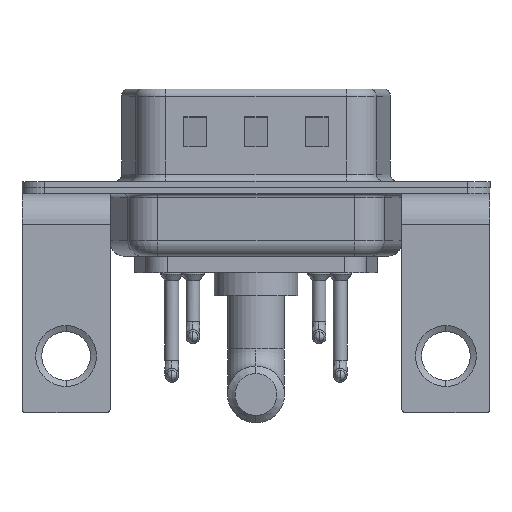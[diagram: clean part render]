
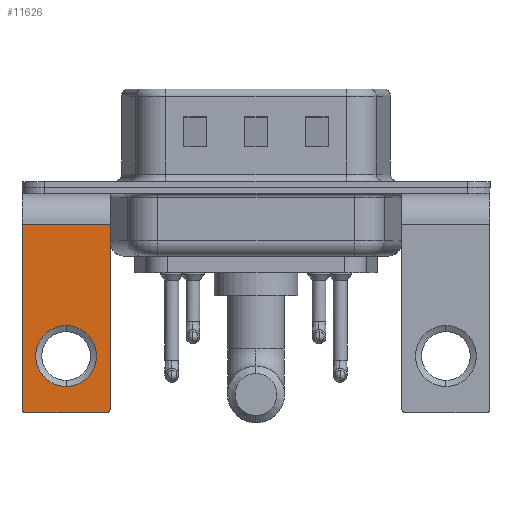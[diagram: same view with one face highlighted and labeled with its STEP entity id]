
A CAD part, front view. The second image highlights one B-rep face of the part: STEP entity #11626.
In plain terms, the highlighted planar face has unit normal (0, -1, 0).
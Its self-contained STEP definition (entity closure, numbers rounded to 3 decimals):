
#47 = EDGE_CURVE ( 'NONE', #15634, #13365, #19505, .T. ) ;
#176 = EDGE_CURVE ( 'NONE', #12546, #8315, #11063, .T. ) ;
#323 = ORIENTED_EDGE ( 'NONE', *, *, #14490, .F. ) ;
#403 = DIRECTION ( 'NONE',  ( 0., 0., 1. ) ) ;
#641 = DIRECTION ( 'NONE',  ( 0., 0., 1. ) ) ;
#1156 = AXIS2_PLACEMENT_3D ( 'NONE', #2812, #17855, #3937 ) ;
#1226 = PLANE ( 'NONE',  #7671 ) ;
#1314 = ORIENTED_EDGE ( 'NONE', *, *, #11258, .T. ) ;
#1354 = CARTESIAN_POINT ( 'NONE',  ( 0., -6.25, -9.07 ) ) ;
#2005 = CARTESIAN_POINT ( 'NONE',  ( 2.9, -6.25, -14.55 ) ) ;
#2027 = LINE ( 'NONE', #19199, #3482 ) ;
#2284 = VERTEX_POINT ( 'NONE', #2005 ) ;
#2810 = CIRCLE ( 'NONE', #13522, 0.25 ) ;
#2812 = CARTESIAN_POINT ( 'NONE',  ( -2.65, -6.25, -14.55 ) ) ;
#3482 = VECTOR ( 'NONE', #14422, 1000. ) ;
#3597 = AXIS2_PLACEMENT_3D ( 'NONE', #4657, #6186, #15428 ) ;
#3713 = ORIENTED_EDGE ( 'NONE', *, *, #7569, .T. ) ;
#3909 = DIRECTION ( 'NONE',  ( 0., -1., 0. ) ) ;
#3937 = DIRECTION ( 'NONE',  ( 0., 0., 1. ) ) ;
#4463 = CIRCLE ( 'NONE', #5101, 2. ) ;
#4496 = FACE_OUTER_BOUND ( 'NONE', #19787, .T. ) ;
#4657 = CARTESIAN_POINT ( 'NONE',  ( 0., -6.25, -11.07 ) ) ;
#5101 = AXIS2_PLACEMENT_3D ( 'NONE', #17385, #19117, #403 ) ;
#6008 = CARTESIAN_POINT ( 'NONE',  ( 2.9, -6.25, -2.4 ) ) ;
#6186 = DIRECTION ( 'NONE',  ( 0., 1., 0. ) ) ;
#6475 = ORIENTED_EDGE ( 'NONE', *, *, #12479, .T. ) ;
#6580 = CARTESIAN_POINT ( 'NONE',  ( -2.9, -6.25, -2.4 ) ) ;
#7569 = EDGE_CURVE ( 'NONE', #8315, #12546, #4463, .T. ) ;
#7671 = AXIS2_PLACEMENT_3D ( 'NONE', #6008, #20034, #16978 ) ;
#8142 = ORIENTED_EDGE ( 'NONE', *, *, #176, .T. ) ;
#8315 = VERTEX_POINT ( 'NONE', #1354 ) ;
#8559 = CARTESIAN_POINT ( 'NONE',  ( 2.65, -6.25, -14.55 ) ) ;
#9077 = VECTOR ( 'NONE', #20070, 1000. ) ;
#9123 = DIRECTION ( 'NONE',  ( -1., 0., 0. ) ) ;
#9892 = EDGE_LOOP ( 'NONE', ( #8142, #3713 ) ) ;
#10391 = VECTOR ( 'NONE', #9123, 1000. ) ;
#10635 = CARTESIAN_POINT ( 'NONE',  ( 0., -6.25, -13.07 ) ) ;
#11063 = CIRCLE ( 'NONE', #3597, 2. ) ;
#11258 = EDGE_CURVE ( 'NONE', #16188, #15780, #17722, .T. ) ;
#11626 = ADVANCED_FACE ( 'NONE', ( #19921, #4496 ), #1226, .F. ) ;
#12253 = VECTOR ( 'NONE', #12790, 1000. ) ;
#12479 = EDGE_CURVE ( 'NONE', #13365, #16188, #19088, .T. ) ;
#12546 = VERTEX_POINT ( 'NONE', #10635 ) ;
#12790 = DIRECTION ( 'NONE',  ( 0., 0., -1. ) ) ;
#13365 = VERTEX_POINT ( 'NONE', #19898 ) ;
#13379 = CARTESIAN_POINT ( 'NONE',  ( -2.65, -6.25, -14.8 ) ) ;
#13522 = AXIS2_PLACEMENT_3D ( 'NONE', #8559, #3909, #641 ) ;
#13707 = CARTESIAN_POINT ( 'NONE',  ( 2.9, -6.25, -2.4 ) ) ;
#13873 = LINE ( 'NONE', #18546, #9077 ) ;
#14422 = DIRECTION ( 'NONE',  ( -1., 0., 0. ) ) ;
#14490 = EDGE_CURVE ( 'NONE', #15634, #2284, #13873, .T. ) ;
#15428 = DIRECTION ( 'NONE',  ( 0., 0., 1. ) ) ;
#15435 = ORIENTED_EDGE ( 'NONE', *, *, #47, .T. ) ;
#15634 = VERTEX_POINT ( 'NONE', #16015 ) ;
#15780 = VERTEX_POINT ( 'NONE', #13379 ) ;
#16015 = CARTESIAN_POINT ( 'NONE',  ( 2.9, -6.25, -2.4 ) ) ;
#16188 = VERTEX_POINT ( 'NONE', #18009 ) ;
#16241 = ORIENTED_EDGE ( 'NONE', *, *, #19968, .F. ) ;
#16978 = DIRECTION ( 'NONE',  ( 0., 0., 1. ) ) ;
#17252 = VERTEX_POINT ( 'NONE', #18242 ) ;
#17385 = CARTESIAN_POINT ( 'NONE',  ( 0., -6.25, -11.07 ) ) ;
#17673 = EDGE_CURVE ( 'NONE', #17252, #2284, #2810, .T. ) ;
#17722 = CIRCLE ( 'NONE', #1156, 0.25 ) ;
#17855 = DIRECTION ( 'NONE',  ( 0., -1., 0. ) ) ;
#18009 = CARTESIAN_POINT ( 'NONE',  ( -2.9, -6.25, -14.55 ) ) ;
#18242 = CARTESIAN_POINT ( 'NONE',  ( 2.65, -6.25, -14.8 ) ) ;
#18546 = CARTESIAN_POINT ( 'NONE',  ( 2.9, -6.25, -2.4 ) ) ;
#19088 = LINE ( 'NONE', #6580, #12253 ) ;
#19098 = ORIENTED_EDGE ( 'NONE', *, *, #17673, .T. ) ;
#19117 = DIRECTION ( 'NONE',  ( 0., 1., 0. ) ) ;
#19199 = CARTESIAN_POINT ( 'NONE',  ( 2.9, -6.25, -14.8 ) ) ;
#19505 = LINE ( 'NONE', #13707, #10391 ) ;
#19787 = EDGE_LOOP ( 'NONE', ( #6475, #1314, #16241, #19098, #323, #15435 ) ) ;
#19898 = CARTESIAN_POINT ( 'NONE',  ( -2.9, -6.25, -2.4 ) ) ;
#19921 = FACE_BOUND ( 'NONE', #9892, .T. ) ;
#19968 = EDGE_CURVE ( 'NONE', #17252, #15780, #2027, .T. ) ;
#20034 = DIRECTION ( 'NONE',  ( 0., 1., 0. ) ) ;
#20070 = DIRECTION ( 'NONE',  ( 0., 0., -1. ) ) ;
